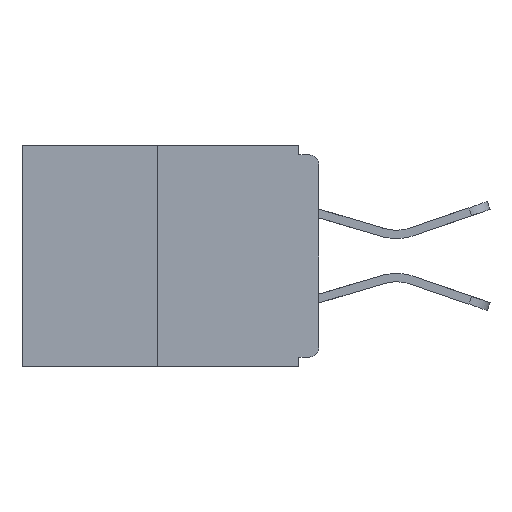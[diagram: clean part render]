
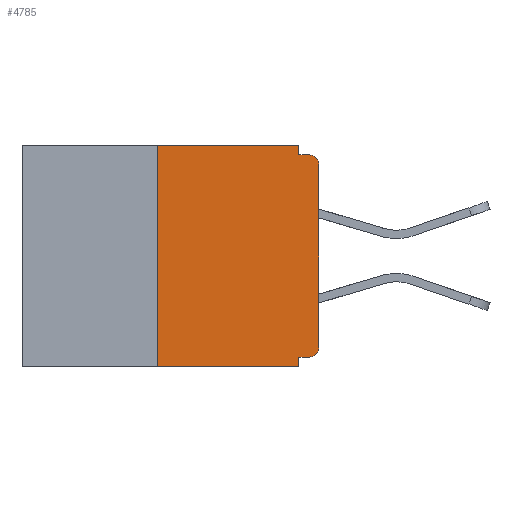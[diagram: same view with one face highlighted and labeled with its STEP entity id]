
A CAD part, left-side view. The second image highlights one B-rep face of the part: STEP entity #4785.
In plain terms, the highlighted planar face has unit normal (-1, 0, 0).
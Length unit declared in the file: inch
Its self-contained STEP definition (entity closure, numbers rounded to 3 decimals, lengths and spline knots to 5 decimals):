
#40 = EDGE_CURVE ( 'NONE', #18170, #5654, #4938, .T. ) ;
#348 = LINE ( 'NONE', #14129, #19329 ) ;
#801 = DIRECTION ( 'NONE',  ( 0., 0., 1. ) ) ;
#1035 = AXIS2_PLACEMENT_3D ( 'NONE', #24646, #11130, #3136 ) ;
#1050 = DIRECTION ( 'NONE',  ( 0., -1., 0. ) ) ;
#1127 = CARTESIAN_POINT ( 'NONE',  ( 0., 0.031, -0.343 ) ) ;
#1505 = EDGE_CURVE ( 'NONE', #20178, #12529, #348, .T. ) ;
#1633 = ORIENTED_EDGE ( 'NONE', *, *, #1505, .T. ) ;
#2767 = LINE ( 'NONE', #3858, #18138 ) ;
#2894 = DIRECTION ( 'NONE',  ( 0., -1., 0. ) ) ;
#3136 = DIRECTION ( 'NONE',  ( 0., 0., -1. ) ) ;
#3224 = FACE_OUTER_BOUND ( 'NONE', #20286, .T. ) ;
#3272 = ORIENTED_EDGE ( 'NONE', *, *, #13899, .F. ) ;
#3527 = LINE ( 'NONE', #8524, #7204 ) ;
#3858 = CARTESIAN_POINT ( 'NONE',  ( 0., 0.031, 0. ) ) ;
#3920 = ORIENTED_EDGE ( 'NONE', *, *, #22189, .F. ) ;
#4037 = ORIENTED_EDGE ( 'NONE', *, *, #19943, .F. ) ;
#4094 = ORIENTED_EDGE ( 'NONE', *, *, #40, .F. ) ;
#4621 = VECTOR ( 'NONE', #14575, 39.37008 ) ;
#4785 = ADVANCED_FACE ( 'NONE', ( #3224 ), #8889, .F. ) ;
#4938 = LINE ( 'NONE', #24253, #4621 ) ;
#5048 = EDGE_CURVE ( 'NONE', #18277, #22643, #8142, .T. ) ;
#5654 = VERTEX_POINT ( 'NONE', #21852 ) ;
#5974 = VECTOR ( 'NONE', #12079, 39.37008 ) ;
#6008 = CARTESIAN_POINT ( 'NONE',  ( 0., 0.25, 0. ) ) ;
#7204 = VECTOR ( 'NONE', #801, 39.37008 ) ;
#7287 = CARTESIAN_POINT ( 'NONE',  ( 0., 0.031, -0.015 ) ) ;
#7352 = VECTOR ( 'NONE', #2894, 39.37008 ) ;
#8142 = LINE ( 'NONE', #23853, #5974 ) ;
#8274 = CARTESIAN_POINT ( 'NONE',  ( 0., 0., -0.313 ) ) ;
#8524 = CARTESIAN_POINT ( 'NONE',  ( 0., 0.25, 0. ) ) ;
#8799 = DIRECTION ( 'NONE',  ( 1., 0., 0. ) ) ;
#8889 = PLANE ( 'NONE',  #11031 ) ;
#9097 = VERTEX_POINT ( 'NONE', #7287 ) ;
#9885 = DIRECTION ( 'NONE',  ( 0., 0., -1. ) ) ;
#10109 = LINE ( 'NONE', #18424, #7352 ) ;
#10633 = ORIENTED_EDGE ( 'NONE', *, *, #16615, .T. ) ;
#10875 = DIRECTION ( 'NONE',  ( 0., 0., -1. ) ) ;
#10908 = CARTESIAN_POINT ( 'NONE',  ( 0., 0.46, -0.343 ) ) ;
#11031 = AXIS2_PLACEMENT_3D ( 'NONE', #24568, #8799, #10875 ) ;
#11130 = DIRECTION ( 'NONE',  ( -1., 0., 0. ) ) ;
#12079 = DIRECTION ( 'NONE',  ( 0., -1., 0. ) ) ;
#12529 = VERTEX_POINT ( 'NONE', #24700 ) ;
#12781 = DIRECTION ( 'NONE',  ( -1., 0., 0. ) ) ;
#13398 = EDGE_CURVE ( 'NONE', #18170, #20178, #13699, .T. ) ;
#13496 = CARTESIAN_POINT ( 'NONE',  ( 0., 0.015, -0.328 ) ) ;
#13699 = CIRCLE ( 'NONE', #1035, 0.015 ) ;
#13899 = EDGE_CURVE ( 'NONE', #19957, #18277, #3527, .T. ) ;
#14129 = CARTESIAN_POINT ( 'NONE',  ( 0., 0., 0. ) ) ;
#14575 = DIRECTION ( 'NONE',  ( 0., 1., 0. ) ) ;
#14988 = DIRECTION ( 'NONE',  ( 0., 0., -1. ) ) ;
#15492 = VECTOR ( 'NONE', #22422, 39.37008 ) ;
#15880 = VECTOR ( 'NONE', #1050, 39.37008 ) ;
#15946 = CIRCLE ( 'NONE', #20140, 0.015 ) ;
#16505 = VERTEX_POINT ( 'NONE', #19659 ) ;
#16615 = EDGE_CURVE ( 'NONE', #12529, #16505, #15946, .T. ) ;
#16791 = CARTESIAN_POINT ( 'NONE',  ( 0., 0.015, -0.03 ) ) ;
#17716 = CARTESIAN_POINT ( 'NONE',  ( 0., 0.25, -0.343 ) ) ;
#18138 = VECTOR ( 'NONE', #9885, 39.37008 ) ;
#18170 = VERTEX_POINT ( 'NONE', #13496 ) ;
#18248 = DIRECTION ( 'NONE',  ( 0., 0., 1. ) ) ;
#18277 = VERTEX_POINT ( 'NONE', #6008 ) ;
#18424 = CARTESIAN_POINT ( 'NONE',  ( 0., 0., -0.015 ) ) ;
#18502 = EDGE_CURVE ( 'NONE', #19957, #19289, #19858, .T. ) ;
#19280 = EDGE_CURVE ( 'NONE', #22643, #9097, #2767, .T. ) ;
#19289 = VERTEX_POINT ( 'NONE', #23247 ) ;
#19329 = VECTOR ( 'NONE', #18248, 39.37008 ) ;
#19659 = CARTESIAN_POINT ( 'NONE',  ( 0., 0.015, -0.015 ) ) ;
#19858 = LINE ( 'NONE', #10908, #15880 ) ;
#19943 = EDGE_CURVE ( 'NONE', #9097, #16505, #10109, .T. ) ;
#19957 = VERTEX_POINT ( 'NONE', #17716 ) ;
#20140 = AXIS2_PLACEMENT_3D ( 'NONE', #16791, #12781, #14988 ) ;
#20178 = VERTEX_POINT ( 'NONE', #8274 ) ;
#20286 = EDGE_LOOP ( 'NONE', ( #20964, #3272, #20566, #3920, #4094, #21601, #1633, #10633, #4037, #23403 ) ) ;
#20566 = ORIENTED_EDGE ( 'NONE', *, *, #18502, .T. ) ;
#20685 = LINE ( 'NONE', #1127, #15492 ) ;
#20964 = ORIENTED_EDGE ( 'NONE', *, *, #5048, .F. ) ;
#21601 = ORIENTED_EDGE ( 'NONE', *, *, #13398, .T. ) ;
#21852 = CARTESIAN_POINT ( 'NONE',  ( 0., 0.031, -0.328 ) ) ;
#22189 = EDGE_CURVE ( 'NONE', #5654, #19289, #20685, .T. ) ;
#22422 = DIRECTION ( 'NONE',  ( 0., 0., -1. ) ) ;
#22643 = VERTEX_POINT ( 'NONE', #22737 ) ;
#22737 = CARTESIAN_POINT ( 'NONE',  ( 0., 0.031, 0. ) ) ;
#23247 = CARTESIAN_POINT ( 'NONE',  ( 0., 0.031, -0.343 ) ) ;
#23403 = ORIENTED_EDGE ( 'NONE', *, *, #19280, .F. ) ;
#23853 = CARTESIAN_POINT ( 'NONE',  ( 0., 0.46, 0. ) ) ;
#24253 = CARTESIAN_POINT ( 'NONE',  ( 0., 0., -0.328 ) ) ;
#24568 = CARTESIAN_POINT ( 'NONE',  ( 0., 0.46, 0. ) ) ;
#24646 = CARTESIAN_POINT ( 'NONE',  ( 0., 0.015, -0.313 ) ) ;
#24700 = CARTESIAN_POINT ( 'NONE',  ( 0., 0., -0.03 ) ) ;
